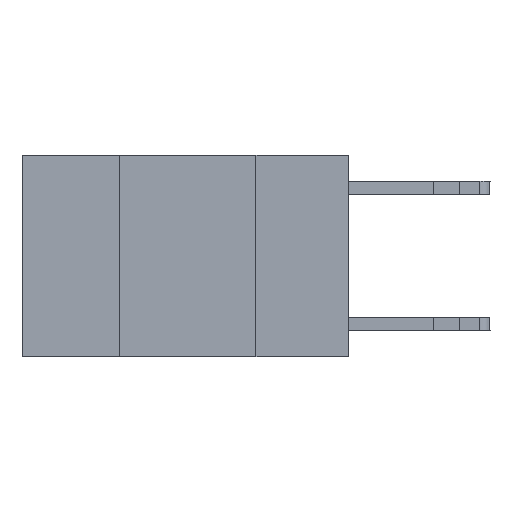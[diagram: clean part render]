
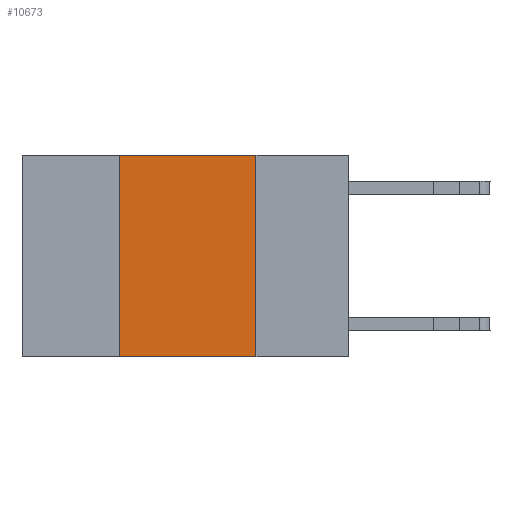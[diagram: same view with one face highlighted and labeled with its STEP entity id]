
A CAD part, left-side view. The second image highlights one B-rep face of the part: STEP entity #10673.
In plain terms, the highlighted planar face has unit normal (-1, 0, 0).
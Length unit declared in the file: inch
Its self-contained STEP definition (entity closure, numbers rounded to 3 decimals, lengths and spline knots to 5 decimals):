
#119 = FACE_OUTER_BOUND ( 'NONE', #2099, .T. ) ;
#122 = VECTOR ( 'NONE', #4054, 39.37008 ) ;
#466 = VECTOR ( 'NONE', #4751, 39.37008 ) ;
#705 = EDGE_CURVE ( 'NONE', #6216, #5519, #10279, .T. ) ;
#834 = AXIS2_PLACEMENT_3D ( 'NONE', #4395, #12770, #6392 ) ;
#941 = ORIENTED_EDGE ( 'NONE', *, *, #6757, .F. ) ;
#966 = DIRECTION ( 'NONE',  ( 0., -1., 0. ) ) ;
#2099 = EDGE_LOOP ( 'NONE', ( #2451, #941, #4608, #8905 ) ) ;
#2230 = PLANE ( 'NONE',  #834 ) ;
#2451 = ORIENTED_EDGE ( 'NONE', *, *, #705, .F. ) ;
#2920 = CARTESIAN_POINT ( 'NONE',  ( 0., 0.6, -0.37 ) ) ;
#3048 = VECTOR ( 'NONE', #966, 39.37008 ) ;
#3187 = LINE ( 'NONE', #8401, #466 ) ;
#3277 = VECTOR ( 'NONE', #11304, 39.37008 ) ;
#4054 = DIRECTION ( 'NONE',  ( 0., 0., -1. ) ) ;
#4395 = CARTESIAN_POINT ( 'NONE',  ( 0., 0.6, 0. ) ) ;
#4608 = ORIENTED_EDGE ( 'NONE', *, *, #5200, .F. ) ;
#4751 = DIRECTION ( 'NONE',  ( 0., 0., 1. ) ) ;
#4783 = CARTESIAN_POINT ( 'NONE',  ( 0., 0.17, 0. ) ) ;
#5200 = EDGE_CURVE ( 'NONE', #12900, #8247, #3187, .T. ) ;
#5519 = VERTEX_POINT ( 'NONE', #9646 ) ;
#6216 = VERTEX_POINT ( 'NONE', #4783 ) ;
#6323 = CARTESIAN_POINT ( 'NONE',  ( 0., 0.17, 0. ) ) ;
#6392 = DIRECTION ( 'NONE',  ( 0., 0., -1. ) ) ;
#6757 = EDGE_CURVE ( 'NONE', #8247, #6216, #7223, .T. ) ;
#7223 = LINE ( 'NONE', #13554, #3048 ) ;
#7373 = EDGE_CURVE ( 'NONE', #12900, #5519, #12340, .T. ) ;
#7561 = CARTESIAN_POINT ( 'NONE',  ( 0., 0.42, 0. ) ) ;
#8247 = VERTEX_POINT ( 'NONE', #7561 ) ;
#8401 = CARTESIAN_POINT ( 'NONE',  ( 0., 0.42, 0. ) ) ;
#8905 = ORIENTED_EDGE ( 'NONE', *, *, #7373, .T. ) ;
#9549 = CARTESIAN_POINT ( 'NONE',  ( 0., 0.42, -0.37 ) ) ;
#9646 = CARTESIAN_POINT ( 'NONE',  ( 0., 0.17, -0.37 ) ) ;
#10279 = LINE ( 'NONE', #6323, #122 ) ;
#10673 = ADVANCED_FACE ( 'NONE', ( #119 ), #2230, .F. ) ;
#11304 = DIRECTION ( 'NONE',  ( 0., -1., 0. ) ) ;
#12340 = LINE ( 'NONE', #2920, #3277 ) ;
#12770 = DIRECTION ( 'NONE',  ( 1., 0., 0. ) ) ;
#12900 = VERTEX_POINT ( 'NONE', #9549 ) ;
#13554 = CARTESIAN_POINT ( 'NONE',  ( 0., 0.6, 0. ) ) ;
